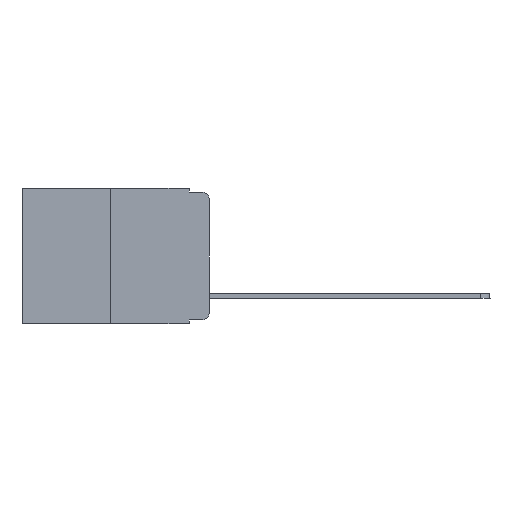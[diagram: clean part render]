
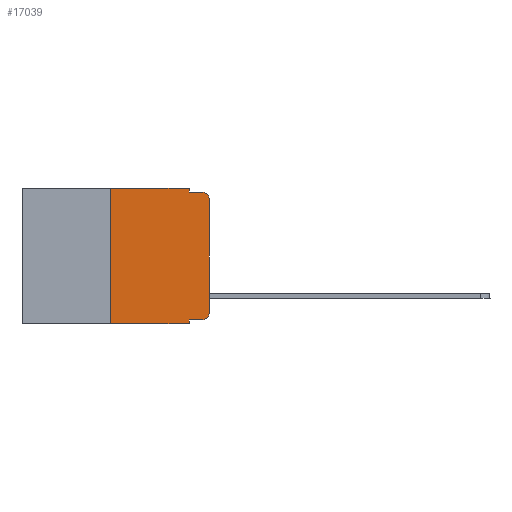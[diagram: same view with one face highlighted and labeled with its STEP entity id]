
A CAD part, left-side view. The second image highlights one B-rep face of the part: STEP entity #17039.
In plain terms, the highlighted planar face has unit normal (-1, 0, 0).
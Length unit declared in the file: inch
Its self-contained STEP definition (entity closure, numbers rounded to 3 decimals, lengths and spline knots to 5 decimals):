
#346 = CARTESIAN_POINT ( 'NONE',  ( 0., 0.051, 0. ) ) ;
#400 = VERTEX_POINT ( 'NONE', #601 ) ;
#519 = ORIENTED_EDGE ( 'NONE', *, *, #19148, .T. ) ;
#601 = CARTESIAN_POINT ( 'NONE',  ( 0., 0.25, 0. ) ) ;
#644 = DIRECTION ( 'NONE',  ( 0., 0., -1. ) ) ;
#677 = CARTESIAN_POINT ( 'NONE',  ( 0., 0.25, 0. ) ) ;
#767 = LINE ( 'NONE', #14094, #16167 ) ;
#1201 = VERTEX_POINT ( 'NONE', #1342 ) ;
#1342 = CARTESIAN_POINT ( 'NONE',  ( 0., 0.051, -0.01 ) ) ;
#1528 = CARTESIAN_POINT ( 'NONE',  ( 0., 0.473, 0. ) ) ;
#1884 = AXIS2_PLACEMENT_3D ( 'NONE', #16530, #18046, #10082 ) ;
#1952 = DIRECTION ( 'NONE',  ( 0., -1., 0. ) ) ;
#2096 = CARTESIAN_POINT ( 'NONE',  ( 0., 0.25, -0.343 ) ) ;
#2148 = CARTESIAN_POINT ( 'NONE',  ( 0., 0.02, -0.333 ) ) ;
#2578 = ORIENTED_EDGE ( 'NONE', *, *, #15398, .F. ) ;
#2624 = ORIENTED_EDGE ( 'NONE', *, *, #12450, .T. ) ;
#2729 = LINE ( 'NONE', #16739, #19093 ) ;
#2899 = VERTEX_POINT ( 'NONE', #2148 ) ;
#3248 = ORIENTED_EDGE ( 'NONE', *, *, #10892, .F. ) ;
#4048 = VECTOR ( 'NONE', #11519, 39.37008 ) ;
#4149 = CARTESIAN_POINT ( 'NONE',  ( 0., 0.02, -0.313 ) ) ;
#4553 = CARTESIAN_POINT ( 'NONE',  ( 0., 0.02, -0.01 ) ) ;
#4561 = DIRECTION ( 'NONE',  ( 0., 0., 1. ) ) ;
#4973 = VERTEX_POINT ( 'NONE', #11681 ) ;
#6037 = LINE ( 'NONE', #16314, #8273 ) ;
#6126 = VERTEX_POINT ( 'NONE', #8581 ) ;
#6608 = CARTESIAN_POINT ( 'NONE',  ( 0., 0.051, -0.01 ) ) ;
#6942 = EDGE_CURVE ( 'NONE', #2899, #4973, #14202, .T. ) ;
#8192 = DIRECTION ( 'NONE',  ( 0., 0., -1. ) ) ;
#8273 = VECTOR ( 'NONE', #11435, 39.37008 ) ;
#8581 = CARTESIAN_POINT ( 'NONE',  ( 0., 0.051, -0.333 ) ) ;
#8939 = DIRECTION ( 'NONE',  ( -1., 0., 0. ) ) ;
#8964 = CARTESIAN_POINT ( 'NONE',  ( 0., 0., -0.03 ) ) ;
#9241 = EDGE_CURVE ( 'NONE', #17490, #1201, #2729, .T. ) ;
#9597 = PLANE ( 'NONE',  #10080 ) ;
#9774 = ORIENTED_EDGE ( 'NONE', *, *, #19723, .F. ) ;
#9796 = AXIS2_PLACEMENT_3D ( 'NONE', #4149, #8939, #644 ) ;
#9905 = LINE ( 'NONE', #18524, #13071 ) ;
#10080 = AXIS2_PLACEMENT_3D ( 'NONE', #1528, #12741, #8192 ) ;
#10082 = DIRECTION ( 'NONE',  ( 0., 0., -1. ) ) ;
#10705 = ORIENTED_EDGE ( 'NONE', *, *, #14523, .F. ) ;
#10775 = CARTESIAN_POINT ( 'NONE',  ( 0., 0.051, -0.343 ) ) ;
#10892 = EDGE_CURVE ( 'NONE', #400, #17490, #16319, .T. ) ;
#10930 = LINE ( 'NONE', #6608, #20349 ) ;
#11435 = DIRECTION ( 'NONE',  ( 0., -1., 0. ) ) ;
#11519 = DIRECTION ( 'NONE',  ( 0., 0., -1. ) ) ;
#11681 = CARTESIAN_POINT ( 'NONE',  ( 0., 0., -0.313 ) ) ;
#11826 = ORIENTED_EDGE ( 'NONE', *, *, #9241, .F. ) ;
#11878 = VERTEX_POINT ( 'NONE', #8964 ) ;
#12450 = EDGE_CURVE ( 'NONE', #11878, #16317, #14265, .T. ) ;
#12650 = VECTOR ( 'NONE', #19840, 39.37008 ) ;
#12741 = DIRECTION ( 'NONE',  ( 1., 0., 0. ) ) ;
#12976 = FACE_OUTER_BOUND ( 'NONE', #16161, .T. ) ;
#13071 = VECTOR ( 'NONE', #19836, 39.37008 ) ;
#13426 = DIRECTION ( 'NONE',  ( 0., 0., -1. ) ) ;
#13646 = LINE ( 'NONE', #677, #12650 ) ;
#14094 = CARTESIAN_POINT ( 'NONE',  ( 0., 0., 0. ) ) ;
#14202 = CIRCLE ( 'NONE', #9796, 0.02 ) ;
#14265 = CIRCLE ( 'NONE', #1884, 0.02 ) ;
#14291 = DIRECTION ( 'NONE',  ( 0., -1., 0. ) ) ;
#14523 = EDGE_CURVE ( 'NONE', #6126, #15008, #19918, .T. ) ;
#15008 = VERTEX_POINT ( 'NONE', #10775 ) ;
#15398 = EDGE_CURVE ( 'NONE', #16602, #400, #13646, .T. ) ;
#16062 = CARTESIAN_POINT ( 'NONE',  ( 0., 0.473, 0. ) ) ;
#16129 = ORIENTED_EDGE ( 'NONE', *, *, #20184, .T. ) ;
#16161 = EDGE_LOOP ( 'NONE', ( #519, #2624, #9774, #11826, #3248, #2578, #16129, #10705, #16594, #17160 ) ) ;
#16167 = VECTOR ( 'NONE', #4561, 39.37008 ) ;
#16200 = CARTESIAN_POINT ( 'NONE',  ( 0., 0.051, 0. ) ) ;
#16314 = CARTESIAN_POINT ( 'NONE',  ( 0., 0.051, -0.333 ) ) ;
#16317 = VERTEX_POINT ( 'NONE', #4553 ) ;
#16319 = LINE ( 'NONE', #16062, #17071 ) ;
#16530 = CARTESIAN_POINT ( 'NONE',  ( 0., 0.02, -0.03 ) ) ;
#16594 = ORIENTED_EDGE ( 'NONE', *, *, #18153, .T. ) ;
#16602 = VERTEX_POINT ( 'NONE', #2096 ) ;
#16739 = CARTESIAN_POINT ( 'NONE',  ( 0., 0.051, 0. ) ) ;
#17039 = ADVANCED_FACE ( 'NONE', ( #12976 ), #9597, .F. ) ;
#17071 = VECTOR ( 'NONE', #14291, 39.37008 ) ;
#17160 = ORIENTED_EDGE ( 'NONE', *, *, #6942, .T. ) ;
#17490 = VERTEX_POINT ( 'NONE', #16200 ) ;
#18046 = DIRECTION ( 'NONE',  ( -1., 0., 0. ) ) ;
#18153 = EDGE_CURVE ( 'NONE', #6126, #2899, #6037, .T. ) ;
#18524 = CARTESIAN_POINT ( 'NONE',  ( 0., 0.473, -0.343 ) ) ;
#19093 = VECTOR ( 'NONE', #13426, 39.37008 ) ;
#19148 = EDGE_CURVE ( 'NONE', #4973, #11878, #767, .T. ) ;
#19723 = EDGE_CURVE ( 'NONE', #1201, #16317, #10930, .T. ) ;
#19836 = DIRECTION ( 'NONE',  ( 0., -1., 0. ) ) ;
#19840 = DIRECTION ( 'NONE',  ( 0., 0., 1. ) ) ;
#19918 = LINE ( 'NONE', #346, #4048 ) ;
#20184 = EDGE_CURVE ( 'NONE', #16602, #15008, #9905, .T. ) ;
#20349 = VECTOR ( 'NONE', #1952, 39.37008 ) ;
